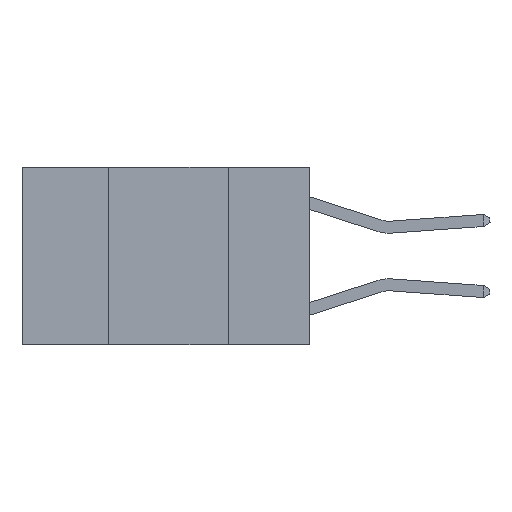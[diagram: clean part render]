
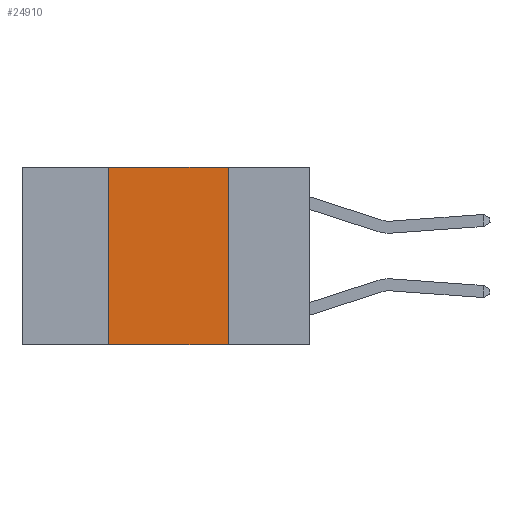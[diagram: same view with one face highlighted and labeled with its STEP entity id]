
A CAD part, left-side view. The second image highlights one B-rep face of the part: STEP entity #24910.
In plain terms, the highlighted planar face has unit normal (-1, 0, 0).
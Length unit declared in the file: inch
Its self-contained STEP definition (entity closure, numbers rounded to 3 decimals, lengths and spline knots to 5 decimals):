
#54 = DIRECTION ( 'NONE',  ( 0., 0., -1. ) ) ;
#949 = VERTEX_POINT ( 'NONE', #7879 ) ;
#970 = CARTESIAN_POINT ( 'NONE',  ( 0., 0.42, 0. ) ) ;
#1267 = PLANE ( 'NONE',  #27970 ) ;
#1576 = LINE ( 'NONE', #970, #4731 ) ;
#2254 = ORIENTED_EDGE ( 'NONE', *, *, #26312, .F. ) ;
#2286 = LINE ( 'NONE', #16314, #8586 ) ;
#3833 = VERTEX_POINT ( 'NONE', #13531 ) ;
#4731 = VECTOR ( 'NONE', #19810, 39.37008 ) ;
#5053 = EDGE_CURVE ( 'NONE', #949, #3833, #2286, .T. ) ;
#6182 = ORIENTED_EDGE ( 'NONE', *, *, #23614, .T. ) ;
#6237 = FACE_OUTER_BOUND ( 'NONE', #30245, .T. ) ;
#6831 = VERTEX_POINT ( 'NONE', #20950 ) ;
#7879 = CARTESIAN_POINT ( 'NONE',  ( 0., 0.42, 0. ) ) ;
#8274 = DIRECTION ( 'NONE',  ( 0., -1., 0. ) ) ;
#8586 = VECTOR ( 'NONE', #21286, 39.37008 ) ;
#10618 = CARTESIAN_POINT ( 'NONE',  ( 0., 0.42, -0.37 ) ) ;
#13259 = CARTESIAN_POINT ( 'NONE',  ( 0., 0.6, 0. ) ) ;
#13531 = CARTESIAN_POINT ( 'NONE',  ( 0., 0.17, 0. ) ) ;
#14619 = VECTOR ( 'NONE', #54, 39.37008 ) ;
#16314 = CARTESIAN_POINT ( 'NONE',  ( 0., 0.6, 0. ) ) ;
#16400 = EDGE_CURVE ( 'NONE', #26529, #949, #1576, .T. ) ;
#17507 = VECTOR ( 'NONE', #8274, 39.37008 ) ;
#19034 = LINE ( 'NONE', #26019, #14619 ) ;
#19804 = DIRECTION ( 'NONE',  ( 1., 0., 0. ) ) ;
#19810 = DIRECTION ( 'NONE',  ( 0., 0., 1. ) ) ;
#20592 = ORIENTED_EDGE ( 'NONE', *, *, #5053, .F. ) ;
#20950 = CARTESIAN_POINT ( 'NONE',  ( 0., 0.17, -0.37 ) ) ;
#21286 = DIRECTION ( 'NONE',  ( 0., -1., 0. ) ) ;
#21878 = ORIENTED_EDGE ( 'NONE', *, *, #16400, .F. ) ;
#22136 = CARTESIAN_POINT ( 'NONE',  ( 0., 0.6, -0.37 ) ) ;
#23614 = EDGE_CURVE ( 'NONE', #26529, #6831, #29560, .T. ) ;
#24910 = ADVANCED_FACE ( 'NONE', ( #6237 ), #1267, .F. ) ;
#26019 = CARTESIAN_POINT ( 'NONE',  ( 0., 0.17, 0. ) ) ;
#26312 = EDGE_CURVE ( 'NONE', #3833, #6831, #19034, .T. ) ;
#26529 = VERTEX_POINT ( 'NONE', #10618 ) ;
#27390 = DIRECTION ( 'NONE',  ( 0., 0., -1. ) ) ;
#27970 = AXIS2_PLACEMENT_3D ( 'NONE', #13259, #19804, #27390 ) ;
#29560 = LINE ( 'NONE', #22136, #17507 ) ;
#30245 = EDGE_LOOP ( 'NONE', ( #2254, #20592, #21878, #6182 ) ) ;
